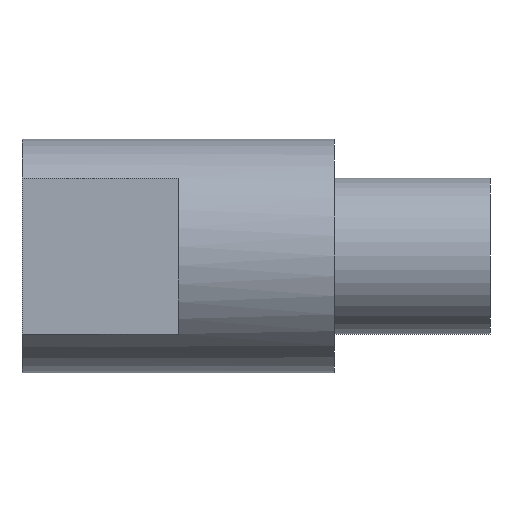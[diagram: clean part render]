
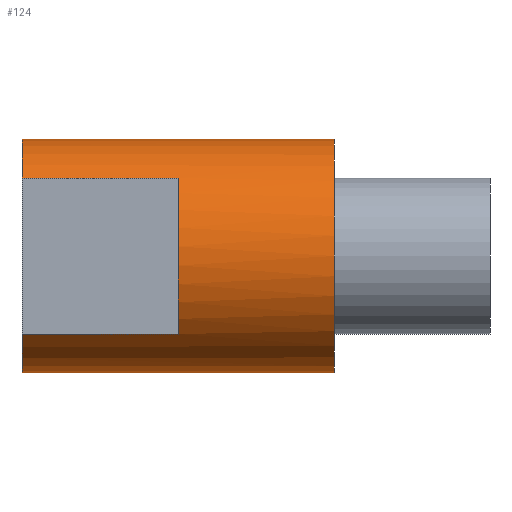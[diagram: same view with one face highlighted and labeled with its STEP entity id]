
A CAD part, left-side view. The second image highlights one B-rep face of the part: STEP entity #124.
In plain terms, the highlighted cylindrical face has radius 7.5 mm (diameter 15 mm), a partial arc.
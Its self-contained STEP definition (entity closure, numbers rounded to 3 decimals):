
#7 = CARTESIAN_POINT ( 'NONE',  ( 0., 20., -7.5 ) ) ;
#15 = VERTEX_POINT ( 'NONE', #176 ) ;
#18 = CARTESIAN_POINT ( 'NONE',  ( 0., 20., 0. ) ) ;
#22 = DIRECTION ( 'NONE',  ( 0., -1., 0. ) ) ;
#23 = DIRECTION ( 'NONE',  ( 0., -1., 0. ) ) ;
#47 = CIRCLE ( 'NONE', #370, 7.5 ) ;
#63 = ORIENTED_EDGE ( 'NONE', *, *, #264, .F. ) ;
#65 = LINE ( 'NONE', #388, #437 ) ;
#72 = CIRCLE ( 'NONE', #377, 7.5 ) ;
#80 = EDGE_LOOP ( 'NONE', ( #466, #475, #301, #336, #283, #63, #477, #233 ) ) ;
#102 = VERTEX_POINT ( 'NONE', #270 ) ;
#103 = AXIS2_PLACEMENT_3D ( 'NONE', #474, #470, #472 ) ;
#108 = CARTESIAN_POINT ( 'NONE',  ( -5.59, 10., 5. ) ) ;
#124 = ADVANCED_FACE ( 'NONE', ( #367 ), #298, .T. ) ;
#129 = LINE ( 'NONE', #285, #348 ) ;
#132 = CARTESIAN_POINT ( 'NONE',  ( 0., 20., 7.5 ) ) ;
#176 = CARTESIAN_POINT ( 'NONE',  ( 0., 0., 7.5 ) ) ;
#182 = CARTESIAN_POINT ( 'NONE',  ( -5.59, 20., -5. ) ) ;
#197 = CARTESIAN_POINT ( 'NONE',  ( 0., 20., -7.5 ) ) ;
#214 = VERTEX_POINT ( 'NONE', #182 ) ;
#217 = VERTEX_POINT ( 'NONE', #305 ) ;
#231 = DIRECTION ( 'NONE',  ( 0., 0., 1. ) ) ;
#233 = ORIENTED_EDGE ( 'NONE', *, *, #257, .T. ) ;
#245 = CIRCLE ( 'NONE', #364, 7.5 ) ;
#247 = VERTEX_POINT ( 'NONE', #197 ) ;
#257 = EDGE_CURVE ( 'NONE', #300, #15, #72, .T. ) ;
#258 = CIRCLE ( 'NONE', #103, 7.5 ) ;
#264 = EDGE_CURVE ( 'NONE', #247, #214, #47, .T. ) ;
#265 = EDGE_CURVE ( 'NONE', #217, #214, #129, .T. ) ;
#266 = EDGE_CURVE ( 'NONE', #325, #217, #245, .T. ) ;
#270 = CARTESIAN_POINT ( 'NONE',  ( -5.59, 20., 5. ) ) ;
#275 = EDGE_CURVE ( 'NONE', #102, #325, #65, .T. ) ;
#277 = EDGE_CURVE ( 'NONE', #102, #401, #258, .T. ) ;
#282 = DIRECTION ( 'NONE',  ( 0., 1., 0. ) ) ;
#283 = ORIENTED_EDGE ( 'NONE', *, *, #265, .T. ) ;
#285 = CARTESIAN_POINT ( 'NONE',  ( -5.59, 20., -5. ) ) ;
#298 = CYLINDRICAL_SURFACE ( 'NONE', #407, 7.5 ) ;
#300 = VERTEX_POINT ( 'NONE', #473 ) ;
#301 = ORIENTED_EDGE ( 'NONE', *, *, #275, .T. ) ;
#305 = CARTESIAN_POINT ( 'NONE',  ( -5.59, 10., -5. ) ) ;
#306 = EDGE_CURVE ( 'NONE', #247, #300, #421, .T. ) ;
#322 = EDGE_CURVE ( 'NONE', #401, #15, #486, .T. ) ;
#325 = VERTEX_POINT ( 'NONE', #108 ) ;
#336 = ORIENTED_EDGE ( 'NONE', *, *, #266, .T. ) ;
#348 = VECTOR ( 'NONE', #282, 1000. ) ;
#364 = AXIS2_PLACEMENT_3D ( 'NONE', #456, #478, #479 ) ;
#367 = FACE_OUTER_BOUND ( 'NONE', #80, .T. ) ;
#369 = DIRECTION ( 'NONE',  ( 0., 1., 0. ) ) ;
#370 = AXIS2_PLACEMENT_3D ( 'NONE', #417, #436, #439 ) ;
#372 = CARTESIAN_POINT ( 'NONE',  ( 0., 20., 7.5 ) ) ;
#375 = DIRECTION ( 'NONE',  ( 0., -1., 0. ) ) ;
#377 = AXIS2_PLACEMENT_3D ( 'NONE', #403, #369, #231 ) ;
#379 = DIRECTION ( 'NONE',  ( 0., -1., 0. ) ) ;
#383 = VECTOR ( 'NONE', #23, 1000. ) ;
#388 = CARTESIAN_POINT ( 'NONE',  ( -5.59, 20., 5. ) ) ;
#401 = VERTEX_POINT ( 'NONE', #372 ) ;
#403 = CARTESIAN_POINT ( 'NONE',  ( 0., 0., 0. ) ) ;
#407 = AXIS2_PLACEMENT_3D ( 'NONE', #18, #375, #420 ) ;
#417 = CARTESIAN_POINT ( 'NONE',  ( 0., 20., 0. ) ) ;
#420 = DIRECTION ( 'NONE',  ( 0., 0., -1. ) ) ;
#421 = LINE ( 'NONE', #7, #458 ) ;
#436 = DIRECTION ( 'NONE',  ( 0., 1., 0. ) ) ;
#437 = VECTOR ( 'NONE', #379, 1000. ) ;
#439 = DIRECTION ( 'NONE',  ( 0., 0., 1. ) ) ;
#456 = CARTESIAN_POINT ( 'NONE',  ( 0., 10., 0. ) ) ;
#458 = VECTOR ( 'NONE', #22, 1000. ) ;
#466 = ORIENTED_EDGE ( 'NONE', *, *, #322, .F. ) ;
#470 = DIRECTION ( 'NONE',  ( 0., 1., 0. ) ) ;
#472 = DIRECTION ( 'NONE',  ( 0., 0., 1. ) ) ;
#473 = CARTESIAN_POINT ( 'NONE',  ( 0., 0., -7.5 ) ) ;
#474 = CARTESIAN_POINT ( 'NONE',  ( 0., 20., 0. ) ) ;
#475 = ORIENTED_EDGE ( 'NONE', *, *, #277, .F. ) ;
#477 = ORIENTED_EDGE ( 'NONE', *, *, #306, .T. ) ;
#478 = DIRECTION ( 'NONE',  ( 0., -1., 0. ) ) ;
#479 = DIRECTION ( 'NONE',  ( 0., 0., -1. ) ) ;
#486 = LINE ( 'NONE', #132, #383 ) ;
